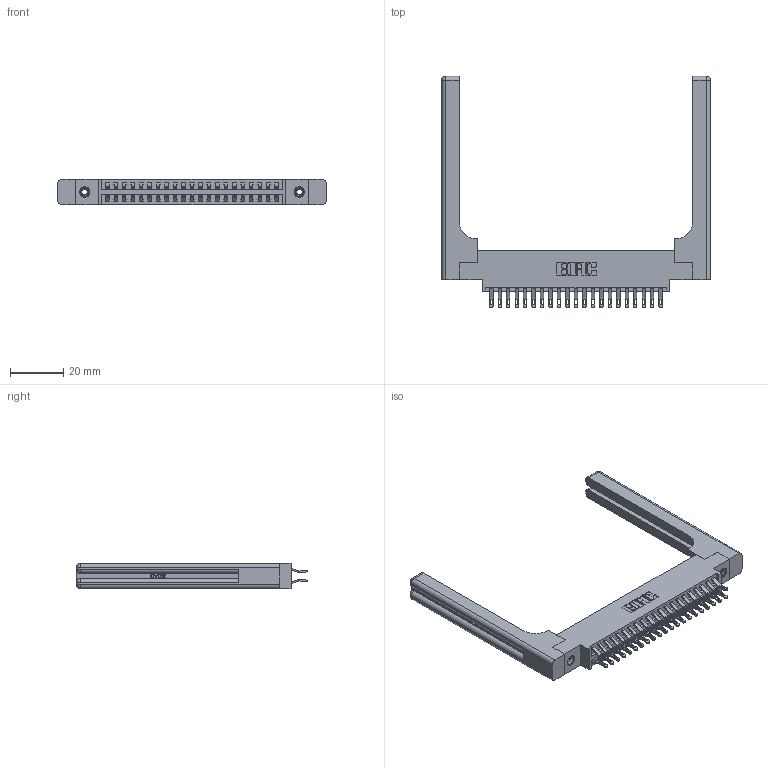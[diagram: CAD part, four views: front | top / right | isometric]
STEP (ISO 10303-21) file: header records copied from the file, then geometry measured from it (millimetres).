
FILE_DESCRIPTION (( 'STEP AP203' ), '1' );
FILE_NAME ('346-042-555-858.STEP', '2022-05-20T05:02:49', ( '' ), ( '' ), 'SwSTEP 2.0', 'SolidWorks 2020', '' );
FILE_SCHEMA (( 'CONFIG_CONTROL_DESIGN' ));
Length unit declared in the file: inch
Products named in the file (5): 346-220-058_345-220-058; 346 Part_0.170 Offset - 0.156 Dia-TH; 345-292-001_555 Tail; 346-042-555-858; 345-250-001_345-250-001-102
Assembly tree (47 placements, depth 2):
  346-042-555-858
    346 Part_0.170 Offset - 0.156 Dia-TH
    345-292-001_555 Tail  x42
    345-250-001_345-250-001-102  x2
    346-220-058_345-220-058  x2
Bounding box: 100.74 x 86.74 x 9.4 mm (x, y, z)
Volume: 17103.3 mm3; surface area: 18499.4 mm2
Topology: 47 solids, 47 shells, 2832 faces, 8729 edges, 5798 vertices
Faces by surface type: plane 1628, cylinder 1144, bspline 36, cone 12, sphere 8, torus 4
Entity records: 22588 total; most frequent: CARTESIAN_POINT 4801, ORIENTED_EDGE 3500, DIRECTION 3182, EDGE_CURVE 1750, LINE 1422, VECTOR 1422, VERTEX_POINT 1158, AXIS2_PLACEMENT_3D 880
